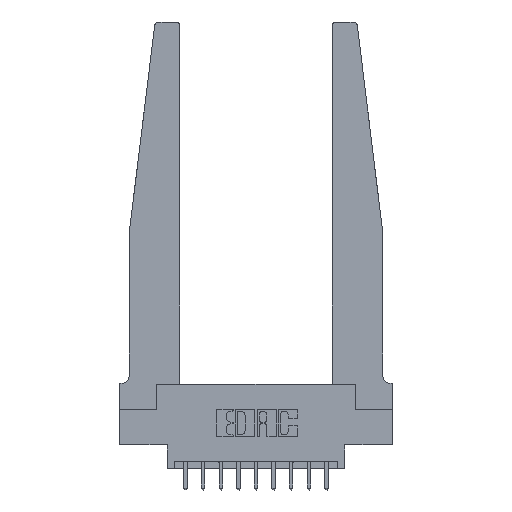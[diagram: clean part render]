
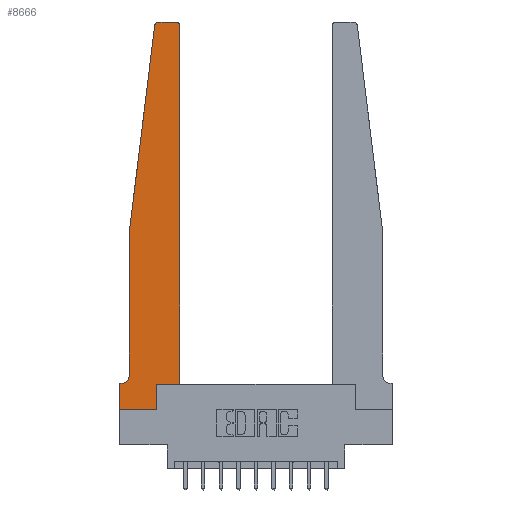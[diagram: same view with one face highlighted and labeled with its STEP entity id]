
A CAD part, top view. The second image highlights one B-rep face of the part: STEP entity #8666.
In plain terms, the highlighted planar face has unit normal (0, 0, 1).
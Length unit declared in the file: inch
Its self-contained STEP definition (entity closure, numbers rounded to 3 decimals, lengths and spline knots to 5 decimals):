
#271 = DIRECTION ( 'NONE',  ( 0., 0., 1. ) ) ;
#594 = LINE ( 'NONE', #753, #3080 ) ;
#703 = VERTEX_POINT ( 'NONE', #12660 ) ;
#753 = CARTESIAN_POINT ( 'NONE',  ( 0., 0., 0.37 ) ) ;
#808 = CARTESIAN_POINT ( 'NONE',  ( 0.27653, 2.72, 0.37 ) ) ;
#903 = LINE ( 'NONE', #3453, #2678 ) ;
#950 = LINE ( 'NONE', #1018, #8371 ) ;
#1018 = CARTESIAN_POINT ( 'NONE',  ( 0.065, 1.25, 0.37 ) ) ;
#1213 = ORIENTED_EDGE ( 'NONE', *, *, #3055, .T. ) ;
#1581 = VECTOR ( 'NONE', #15559, 39.37008 ) ;
#1825 = AXIS2_PLACEMENT_3D ( 'NONE', #14991, #5390, #3523 ) ;
#1946 = DIRECTION ( 'NONE',  ( 0., 1., 0. ) ) ;
#2027 = DIRECTION ( 'NONE',  ( 1., 0., 0. ) ) ;
#2171 = AXIS2_PLACEMENT_3D ( 'NONE', #9227, #2503, #2027 ) ;
#2354 = DIRECTION ( 'NONE',  ( 0., 1., 0. ) ) ;
#2503 = DIRECTION ( 'NONE',  ( 0., 0., 1. ) ) ;
#2656 = VECTOR ( 'NONE', #11306, 39.37008 ) ;
#2678 = VECTOR ( 'NONE', #1946, 39.37008 ) ;
#2860 = CARTESIAN_POINT ( 'NONE',  ( 0.25, 2.75, 0.37 ) ) ;
#3055 = EDGE_CURVE ( 'NONE', #703, #15518, #15161, .T. ) ;
#3080 = VECTOR ( 'NONE', #5419, 39.37008 ) ;
#3307 = VERTEX_POINT ( 'NONE', #10641 ) ;
#3453 = CARTESIAN_POINT ( 'NONE',  ( 0.425, 0.18, 0.37 ) ) ;
#3474 = VECTOR ( 'NONE', #12683, 39.37008 ) ;
#3523 = DIRECTION ( 'NONE',  ( -1., 0., 0. ) ) ;
#3691 = CARTESIAN_POINT ( 'NONE',  ( 0.2605, 0.18, 0.37 ) ) ;
#3720 = EDGE_CURVE ( 'NONE', #7558, #14679, #8644, .T. ) ;
#3742 = EDGE_CURVE ( 'NONE', #9617, #3307, #10440, .T. ) ;
#3947 = CARTESIAN_POINT ( 'NONE',  ( 0.27653, 2.75, 0.37 ) ) ;
#4028 = VERTEX_POINT ( 'NONE', #12281 ) ;
#4376 = LINE ( 'NONE', #11638, #1581 ) ;
#4538 = DIRECTION ( 'NONE',  ( 1., 0., 0. ) ) ;
#4627 = CARTESIAN_POINT ( 'NONE',  ( 0.2605, 0.18, 0.37 ) ) ;
#4673 = EDGE_CURVE ( 'NONE', #4028, #4873, #12918, .T. ) ;
#4708 = CARTESIAN_POINT ( 'NONE',  ( 0.425, 0.18, 0.37 ) ) ;
#4873 = VERTEX_POINT ( 'NONE', #5554 ) ;
#5145 = EDGE_CURVE ( 'NONE', #3307, #10377, #11178, .T. ) ;
#5390 = DIRECTION ( 'NONE',  ( 0., 0., -1. ) ) ;
#5419 = DIRECTION ( 'NONE',  ( 0., -1., 0. ) ) ;
#5554 = CARTESIAN_POINT ( 'NONE',  ( 0.395, 2.75, 0.37 ) ) ;
#5749 = DIRECTION ( 'NONE',  ( 0., -1., 0. ) ) ;
#5769 = ORIENTED_EDGE ( 'NONE', *, *, #11598, .T. ) ;
#5837 = ORIENTED_EDGE ( 'NONE', *, *, #3720, .T. ) ;
#6101 = AXIS2_PLACEMENT_3D ( 'NONE', #6134, #271, #11109 ) ;
#6134 = CARTESIAN_POINT ( 'NONE',  ( 0.395, 2.72, 0.37 ) ) ;
#6162 = LINE ( 'NONE', #2860, #2656 ) ;
#6168 = ORIENTED_EDGE ( 'NONE', *, *, #4673, .T. ) ;
#6813 = ORIENTED_EDGE ( 'NONE', *, *, #7197, .T. ) ;
#7082 = ORIENTED_EDGE ( 'NONE', *, *, #10167, .T. ) ;
#7197 = EDGE_CURVE ( 'NONE', #4873, #9617, #6162, .T. ) ;
#7547 = CARTESIAN_POINT ( 'NONE',  ( 0.065, 1.25, 0.37 ) ) ;
#7558 = VERTEX_POINT ( 'NONE', #9795 ) ;
#7802 = ORIENTED_EDGE ( 'NONE', *, *, #5145, .T. ) ;
#7915 = VERTEX_POINT ( 'NONE', #9538 ) ;
#7928 = EDGE_CURVE ( 'NONE', #15518, #12475, #13346, .T. ) ;
#8371 = VECTOR ( 'NONE', #5749, 39.37008 ) ;
#8644 = CIRCLE ( 'NONE', #1825, 0.05 ) ;
#8666 = ADVANCED_FACE ( 'NONE', ( #9672 ), #12850, .T. ) ;
#8906 = CARTESIAN_POINT ( 'NONE',  ( 0., 0., 0.37 ) ) ;
#9043 = CARTESIAN_POINT ( 'NONE',  ( 0.2605, 0., 0.37 ) ) ;
#9193 = VECTOR ( 'NONE', #4538, 39.37008 ) ;
#9227 = CARTESIAN_POINT ( 'NONE',  ( 0., 0.1875, 0.37 ) ) ;
#9360 = CARTESIAN_POINT ( 'NONE',  ( 0., 0.1875, 0.37 ) ) ;
#9538 = CARTESIAN_POINT ( 'NONE',  ( 0.425, 0.18, 0.37 ) ) ;
#9617 = VERTEX_POINT ( 'NONE', #3947 ) ;
#9661 = VECTOR ( 'NONE', #11332, 39.37008 ) ;
#9672 = FACE_OUTER_BOUND ( 'NONE', #11894, .T. ) ;
#9795 = CARTESIAN_POINT ( 'NONE',  ( 0.065, 0.2375, 0.37 ) ) ;
#10167 = EDGE_CURVE ( 'NONE', #7915, #4028, #903, .T. ) ;
#10377 = VERTEX_POINT ( 'NONE', #13150 ) ;
#10440 = CIRCLE ( 'NONE', #14500, 0.03 ) ;
#10618 = ORIENTED_EDGE ( 'NONE', *, *, #15171, .T. ) ;
#10641 = CARTESIAN_POINT ( 'NONE',  ( 0.24675, 2.72367, 0.37 ) ) ;
#10687 = EDGE_CURVE ( 'NONE', #10377, #7558, #950, .T. ) ;
#11031 = EDGE_CURVE ( 'NONE', #12410, #703, #594, .T. ) ;
#11109 = DIRECTION ( 'NONE',  ( 1., 0., 0. ) ) ;
#11178 = LINE ( 'NONE', #7547, #9661 ) ;
#11306 = DIRECTION ( 'NONE',  ( -1., 0., 0. ) ) ;
#11332 = DIRECTION ( 'NONE',  ( -0.122, -0.992, 0. ) ) ;
#11338 = ORIENTED_EDGE ( 'NONE', *, *, #10687, .T. ) ;
#11598 = EDGE_CURVE ( 'NONE', #14679, #12410, #4376, .T. ) ;
#11633 = DIRECTION ( 'NONE',  ( 1., 0., 0. ) ) ;
#11638 = CARTESIAN_POINT ( 'NONE',  ( 0.065, 0.1875, 0.37 ) ) ;
#11880 = LINE ( 'NONE', #4708, #9193 ) ;
#11894 = EDGE_LOOP ( 'NONE', ( #6813, #12360, #7802, #11338, #5837, #5769, #15483, #1213, #14111, #10618, #7082, #6168 ) ) ;
#12281 = CARTESIAN_POINT ( 'NONE',  ( 0.425, 2.72, 0.37 ) ) ;
#12360 = ORIENTED_EDGE ( 'NONE', *, *, #3742, .T. ) ;
#12410 = VERTEX_POINT ( 'NONE', #9360 ) ;
#12475 = VERTEX_POINT ( 'NONE', #3691 ) ;
#12660 = CARTESIAN_POINT ( 'NONE',  ( 0., 0., 0.37 ) ) ;
#12683 = DIRECTION ( 'NONE',  ( 1., 0., 0. ) ) ;
#12850 = PLANE ( 'NONE',  #2171 ) ;
#12918 = CIRCLE ( 'NONE', #6101, 0.03 ) ;
#13150 = CARTESIAN_POINT ( 'NONE',  ( 0.065, 1.25, 0.37 ) ) ;
#13346 = LINE ( 'NONE', #4627, #15556 ) ;
#14111 = ORIENTED_EDGE ( 'NONE', *, *, #7928, .T. ) ;
#14117 = DIRECTION ( 'NONE',  ( 0., 0., 1. ) ) ;
#14500 = AXIS2_PLACEMENT_3D ( 'NONE', #808, #14117, #11633 ) ;
#14679 = VERTEX_POINT ( 'NONE', #14943 ) ;
#14943 = CARTESIAN_POINT ( 'NONE',  ( 0.015, 0.1875, 0.37 ) ) ;
#14991 = CARTESIAN_POINT ( 'NONE',  ( 0.015, 0.2375, 0.37 ) ) ;
#15161 = LINE ( 'NONE', #8906, #3474 ) ;
#15171 = EDGE_CURVE ( 'NONE', #12475, #7915, #11880, .T. ) ;
#15483 = ORIENTED_EDGE ( 'NONE', *, *, #11031, .T. ) ;
#15518 = VERTEX_POINT ( 'NONE', #9043 ) ;
#15556 = VECTOR ( 'NONE', #2354, 39.37008 ) ;
#15559 = DIRECTION ( 'NONE',  ( -1., 0., 0. ) ) ;
